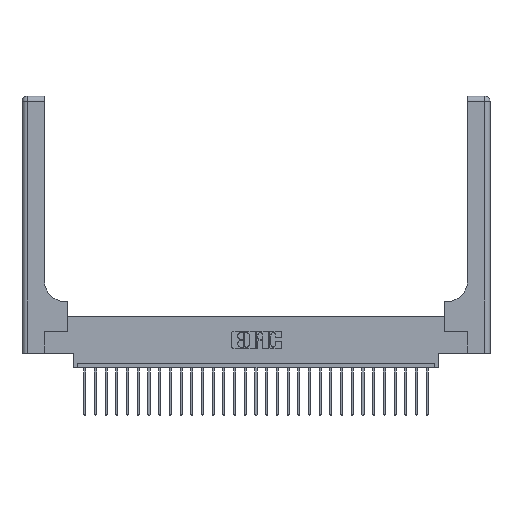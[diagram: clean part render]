
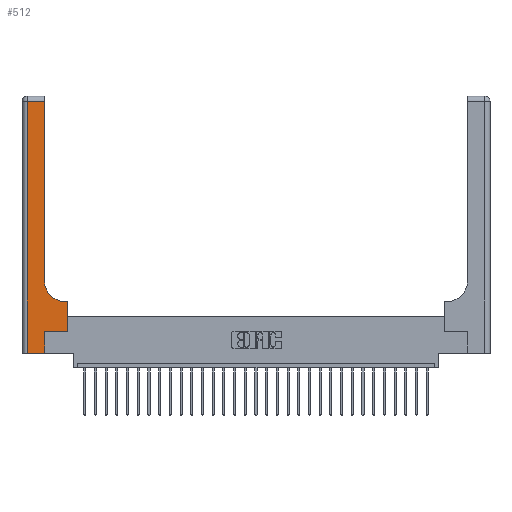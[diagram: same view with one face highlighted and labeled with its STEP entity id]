
A CAD part, top view. The second image highlights one B-rep face of the part: STEP entity #512.
In plain terms, the highlighted planar face has unit normal (0, 0, 1).
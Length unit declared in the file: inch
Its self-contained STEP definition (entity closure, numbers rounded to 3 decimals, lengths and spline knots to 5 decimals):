
#427 = CIRCLE ( 'NONE', #21749, 0.25 ) ;
#512 = ADVANCED_FACE ( 'NONE', ( #26942 ), #14047, .F. ) ;
#707 = EDGE_CURVE ( 'NONE', #8631, #24036, #10227, .T. ) ;
#1246 = DIRECTION ( 'NONE',  ( 0., 0., -1. ) ) ;
#2062 = LINE ( 'NONE', #10565, #19579 ) ;
#2104 = DIRECTION ( 'NONE',  ( 0., 1., 0. ) ) ;
#2239 = VERTEX_POINT ( 'NONE', #4268 ) ;
#2798 = VECTOR ( 'NONE', #21063, 39.37008 ) ;
#3118 = ORIENTED_EDGE ( 'NONE', *, *, #17875, .T. ) ;
#3492 = DIRECTION ( 'NONE',  ( 0., -1., 0. ) ) ;
#3504 = VERTEX_POINT ( 'NONE', #8968 ) ;
#3635 = CARTESIAN_POINT ( 'NONE',  ( 0.06, 3., 0.37 ) ) ;
#3849 = VERTEX_POINT ( 'NONE', #17790 ) ;
#4268 = CARTESIAN_POINT ( 'NONE',  ( 0.528, 0.25, 0.37 ) ) ;
#4433 = EDGE_CURVE ( 'NONE', #24036, #24048, #427, .T. ) ;
#4509 = ORIENTED_EDGE ( 'NONE', *, *, #20238, .T. ) ;
#4595 = DIRECTION ( 'NONE',  ( -1., 0., 0. ) ) ;
#5437 = LINE ( 'NONE', #14033, #12379 ) ;
#5600 = ORIENTED_EDGE ( 'NONE', *, *, #20735, .T. ) ;
#5852 = EDGE_CURVE ( 'NONE', #24048, #14294, #27034, .T. ) ;
#5859 = LINE ( 'NONE', #3635, #21188 ) ;
#6646 = ORIENTED_EDGE ( 'NONE', *, *, #22898, .T. ) ;
#7103 = VECTOR ( 'NONE', #22200, 39.37008 ) ;
#7177 = CARTESIAN_POINT ( 'NONE',  ( 0.51, 0.6, 0.37 ) ) ;
#7964 = DIRECTION ( 'NONE',  ( -1., 0., 0. ) ) ;
#8631 = VERTEX_POINT ( 'NONE', #26201 ) ;
#8746 = VECTOR ( 'NONE', #2104, 39.37008 ) ;
#8968 = CARTESIAN_POINT ( 'NONE',  ( 0.265, 0.25, 0.37 ) ) ;
#9601 = CARTESIAN_POINT ( 'NONE',  ( 0.06, 0., 0.37 ) ) ;
#9708 = DIRECTION ( 'NONE',  ( 0., 1., 0. ) ) ;
#10227 = LINE ( 'NONE', #20652, #2798 ) ;
#10228 = VERTEX_POINT ( 'NONE', #22930 ) ;
#10565 = CARTESIAN_POINT ( 'NONE',  ( 0., 2.94, 0.37 ) ) ;
#11480 = DIRECTION ( 'NONE',  ( 0., 1., 0. ) ) ;
#11583 = CARTESIAN_POINT ( 'NONE',  ( 0.26, 0.85, 0.37 ) ) ;
#12379 = VECTOR ( 'NONE', #20437, 39.37008 ) ;
#13678 = EDGE_CURVE ( 'NONE', #19426, #3849, #5437, .T. ) ;
#13906 = DIRECTION ( 'NONE',  ( 1., 0., 0. ) ) ;
#14033 = CARTESIAN_POINT ( 'NONE',  ( 0., 0., 0.37 ) ) ;
#14034 = DIRECTION ( 'NONE',  ( 0., 0., -1. ) ) ;
#14047 = PLANE ( 'NONE',  #20080 ) ;
#14294 = VERTEX_POINT ( 'NONE', #22899 ) ;
#14870 = ORIENTED_EDGE ( 'NONE', *, *, #4433, .T. ) ;
#15591 = VECTOR ( 'NONE', #9708, 39.37008 ) ;
#15947 = CARTESIAN_POINT ( 'NONE',  ( 0.265, 0.25, 0.37 ) ) ;
#17790 = CARTESIAN_POINT ( 'NONE',  ( 0.265, 0., 0.37 ) ) ;
#17875 = EDGE_CURVE ( 'NONE', #10228, #19426, #5859, .T. ) ;
#18041 = CARTESIAN_POINT ( 'NONE',  ( 0.528, 0.25, 0.37 ) ) ;
#18250 = CARTESIAN_POINT ( 'NONE',  ( 0., 3., 0.37 ) ) ;
#18956 = LINE ( 'NONE', #24903, #8746 ) ;
#18989 = ORIENTED_EDGE ( 'NONE', *, *, #24728, .T. ) ;
#19426 = VERTEX_POINT ( 'NONE', #9601 ) ;
#19579 = VECTOR ( 'NONE', #4595, 39.37008 ) ;
#19821 = ORIENTED_EDGE ( 'NONE', *, *, #707, .T. ) ;
#20080 = AXIS2_PLACEMENT_3D ( 'NONE', #18250, #1246, #7964 ) ;
#20238 = EDGE_CURVE ( 'NONE', #3849, #3504, #18956, .T. ) ;
#20252 = LINE ( 'NONE', #15947, #7103 ) ;
#20437 = DIRECTION ( 'NONE',  ( 1., 0., 0. ) ) ;
#20652 = CARTESIAN_POINT ( 'NONE',  ( 0.26, 0.6, 0.37 ) ) ;
#20735 = EDGE_CURVE ( 'NONE', #3504, #2239, #20252, .T. ) ;
#21063 = DIRECTION ( 'NONE',  ( -1., 0., 0. ) ) ;
#21073 = ORIENTED_EDGE ( 'NONE', *, *, #13678, .T. ) ;
#21188 = VECTOR ( 'NONE', #3492, 39.37008 ) ;
#21749 = AXIS2_PLACEMENT_3D ( 'NONE', #22107, #14034, #13906 ) ;
#22107 = CARTESIAN_POINT ( 'NONE',  ( 0.51, 0.85, 0.37 ) ) ;
#22200 = DIRECTION ( 'NONE',  ( 1., 0., 0. ) ) ;
#22743 = ORIENTED_EDGE ( 'NONE', *, *, #5852, .T. ) ;
#22898 = EDGE_CURVE ( 'NONE', #14294, #10228, #2062, .T. ) ;
#22899 = CARTESIAN_POINT ( 'NONE',  ( 0.26, 2.94, 0.37 ) ) ;
#22930 = CARTESIAN_POINT ( 'NONE',  ( 0.06, 2.94, 0.37 ) ) ;
#24036 = VERTEX_POINT ( 'NONE', #7177 ) ;
#24048 = VERTEX_POINT ( 'NONE', #11583 ) ;
#24261 = LINE ( 'NONE', #18041, #26662 ) ;
#24728 = EDGE_CURVE ( 'NONE', #2239, #8631, #24261, .T. ) ;
#24903 = CARTESIAN_POINT ( 'NONE',  ( 0.265, 0., 0.37 ) ) ;
#25714 = EDGE_LOOP ( 'NONE', ( #22743, #6646, #3118, #21073, #4509, #5600, #18989, #19821, #14870 ) ) ;
#26201 = CARTESIAN_POINT ( 'NONE',  ( 0.528, 0.6, 0.37 ) ) ;
#26662 = VECTOR ( 'NONE', #11480, 39.37008 ) ;
#26893 = CARTESIAN_POINT ( 'NONE',  ( 0.26, 3., 0.37 ) ) ;
#26942 = FACE_OUTER_BOUND ( 'NONE', #25714, .T. ) ;
#27034 = LINE ( 'NONE', #26893, #15591 ) ;
